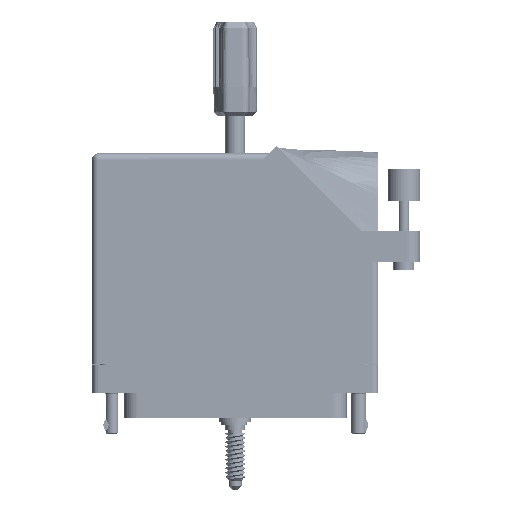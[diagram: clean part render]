
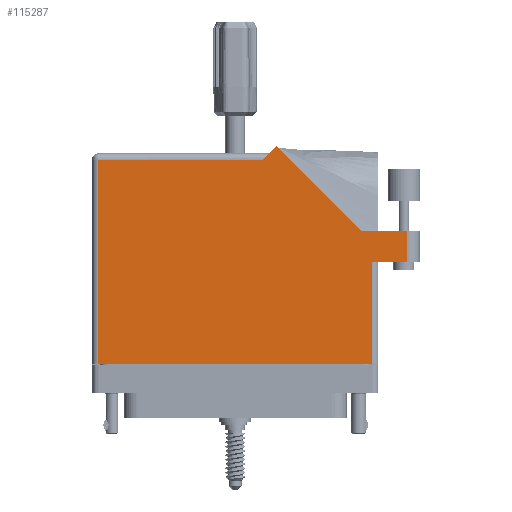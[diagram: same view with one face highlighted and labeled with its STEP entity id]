
A CAD part, front view. The second image highlights one B-rep face of the part: STEP entity #115287.
In plain terms, the highlighted face is planar.
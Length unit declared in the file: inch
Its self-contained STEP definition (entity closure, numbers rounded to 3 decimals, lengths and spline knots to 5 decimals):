
#3873 = ORIENTED_EDGE ( 'NONE', *, *, #112041, .T. ) ;
#5355 = AXIS2_PLACEMENT_3D ( 'NONE', #47061, #21846, #82880 ) ;
#5374 = VECTOR ( 'NONE', #27469, 39.37008 ) ;
#6034 = EDGE_CURVE ( 'NONE', #66235, #62682, #20207, .T. ) ;
#6115 = CARTESIAN_POINT ( 'NONE',  ( -1.3155, 1.868, 0.765 ) ) ;
#6356 = VECTOR ( 'NONE', #63963, 39.37008 ) ;
#6694 = CARTESIAN_POINT ( 'NONE',  ( 1.3775, 0.88, 0.765 ) ) ;
#7200 = LINE ( 'NONE', #78224, #85455 ) ;
#9498 = ORIENTED_EDGE ( 'NONE', *, *, #61071, .T. ) ;
#10416 = DIRECTION ( 'NONE',  ( 0., 1., 0. ) ) ;
#11402 = CARTESIAN_POINT ( 'NONE',  ( -1.3775, -0.1, 0.765 ) ) ;
#11787 = LINE ( 'NONE', #47573, #24042 ) ;
#12413 = DIRECTION ( 'NONE',  ( -1., 0., 0. ) ) ;
#13037 = FACE_OUTER_BOUND ( 'NONE', #88986, .T. ) ;
#17695 = VECTOR ( 'NONE', #91794, 39.37008 ) ;
#18454 = VERTEX_POINT ( 'NONE', #6115 ) ;
#19219 = LINE ( 'NONE', #71476, #5374 ) ;
#20207 = LINE ( 'NONE', #11402, #17695 ) ;
#21846 = DIRECTION ( 'NONE',  ( 0., 0., -1. ) ) ;
#21960 = LINE ( 'NONE', #85326, #41538 ) ;
#22648 = VERTEX_POINT ( 'NONE', #87952 ) ;
#24042 = VECTOR ( 'NONE', #27105, 39.37008 ) ;
#27105 = DIRECTION ( 'NONE',  ( 0., -1., 0. ) ) ;
#27469 = DIRECTION ( 'NONE',  ( -1., 0., 0. ) ) ;
#28581 = ORIENTED_EDGE ( 'NONE', *, *, #6034, .T. ) ;
#33112 = LINE ( 'NONE', #6694, #102352 ) ;
#36075 = CARTESIAN_POINT ( 'NONE',  ( 1.21192, 1.187, 0.765 ) ) ;
#36968 = LINE ( 'NONE', #108542, #6356 ) ;
#41538 = VECTOR ( 'NONE', #47773, 39.37008 ) ;
#41904 = DIRECTION ( 'NONE',  ( 1., 0., 0. ) ) ;
#42681 = VERTEX_POINT ( 'NONE', #66948 ) ;
#44009 = CARTESIAN_POINT ( 'NONE',  ( 0.2655, 1.868, 0.765 ) ) ;
#44721 = DIRECTION ( 'NONE',  ( 0., 1., 0. ) ) ;
#46179 = CARTESIAN_POINT ( 'NONE',  ( 1.3155, 0.88, 0.765 ) ) ;
#47061 = CARTESIAN_POINT ( 'NONE',  ( -1.3775, 1.93, 0.765 ) ) ;
#47573 = CARTESIAN_POINT ( 'NONE',  ( -1.3155, -0.1, 0.765 ) ) ;
#47659 = PLANE ( 'NONE',  #5355 ) ;
#47773 = DIRECTION ( 'NONE',  ( -0.707, -0.707, 0. ) ) ;
#48948 = EDGE_CURVE ( 'NONE', #18454, #66235, #11787, .T. ) ;
#50022 = EDGE_CURVE ( 'NONE', #112417, #18454, #19219, .T. ) ;
#54339 = ORIENTED_EDGE ( 'NONE', *, *, #77755, .T. ) ;
#56014 = EDGE_CURVE ( 'NONE', #22648, #99484, #33112, .T. ) ;
#58530 = ORIENTED_EDGE ( 'NONE', *, *, #75625, .T. ) ;
#60821 = CARTESIAN_POINT ( 'NONE',  ( 1.3155, -0.1, 0.765 ) ) ;
#61071 = EDGE_CURVE ( 'NONE', #62682, #22648, #112333, .T. ) ;
#62682 = VERTEX_POINT ( 'NONE', #60821 ) ;
#63963 = DIRECTION ( 'NONE',  ( -0.707, 0.707, 0. ) ) ;
#66235 = VERTEX_POINT ( 'NONE', #96313 ) ;
#66948 = CARTESIAN_POINT ( 'NONE',  ( 1.6525, 1.187, 0.765 ) ) ;
#70483 = CARTESIAN_POINT ( 'NONE',  ( 1.6525, 0.88, 0.765 ) ) ;
#71064 = CARTESIAN_POINT ( 'NONE',  ( 0.39821, 2.00071, 0.765 ) ) ;
#71476 = CARTESIAN_POINT ( 'NONE',  ( -1.3775, 1.868, 0.765 ) ) ;
#72771 = VECTOR ( 'NONE', #12413, 39.37008 ) ;
#75477 = VERTEX_POINT ( 'NONE', #36075 ) ;
#75625 = EDGE_CURVE ( 'NONE', #99660, #112417, #21960, .T. ) ;
#77755 = EDGE_CURVE ( 'NONE', #75477, #99660, #36968, .T. ) ;
#78224 = CARTESIAN_POINT ( 'NONE',  ( 1.6525, 1.187, 0.765 ) ) ;
#81703 = CARTESIAN_POINT ( 'NONE',  ( 1.7775, 1.187, 0.765 ) ) ;
#82880 = DIRECTION ( 'NONE',  ( -1., 0., 0. ) ) ;
#84828 = ORIENTED_EDGE ( 'NONE', *, *, #95809, .T. ) ;
#85326 = CARTESIAN_POINT ( 'NONE',  ( 0.3275, 1.93, 0.765 ) ) ;
#85455 = VECTOR ( 'NONE', #44721, 39.37008 ) ;
#87728 = ORIENTED_EDGE ( 'NONE', *, *, #48948, .T. ) ;
#87952 = CARTESIAN_POINT ( 'NONE',  ( 1.3155, 0.88, 0.765 ) ) ;
#88986 = EDGE_LOOP ( 'NONE', ( #106504, #3873, #84828, #54339, #58530, #113415, #87728, #28581, #9498 ) ) ;
#90471 = LINE ( 'NONE', #81703, #72771 ) ;
#91691 = VECTOR ( 'NONE', #10416, 39.37008 ) ;
#91794 = DIRECTION ( 'NONE',  ( 1., 0., 0. ) ) ;
#95809 = EDGE_CURVE ( 'NONE', #42681, #75477, #90471, .T. ) ;
#96313 = CARTESIAN_POINT ( 'NONE',  ( -1.3155, -0.1, 0.765 ) ) ;
#99484 = VERTEX_POINT ( 'NONE', #70483 ) ;
#99660 = VERTEX_POINT ( 'NONE', #71064 ) ;
#102352 = VECTOR ( 'NONE', #41904, 39.37008 ) ;
#106504 = ORIENTED_EDGE ( 'NONE', *, *, #56014, .T. ) ;
#108542 = CARTESIAN_POINT ( 'NONE',  ( 1.21192, 1.187, 0.765 ) ) ;
#112041 = EDGE_CURVE ( 'NONE', #99484, #42681, #7200, .T. ) ;
#112333 = LINE ( 'NONE', #46179, #91691 ) ;
#112417 = VERTEX_POINT ( 'NONE', #44009 ) ;
#113415 = ORIENTED_EDGE ( 'NONE', *, *, #50022, .T. ) ;
#115287 = ADVANCED_FACE ( 'NONE', ( #13037 ), #47659, .F. ) ;
